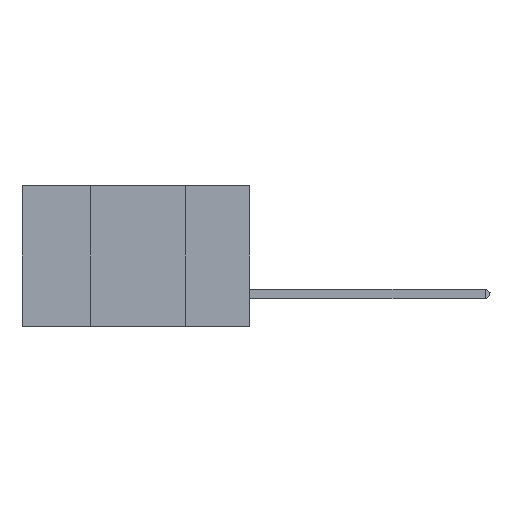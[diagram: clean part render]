
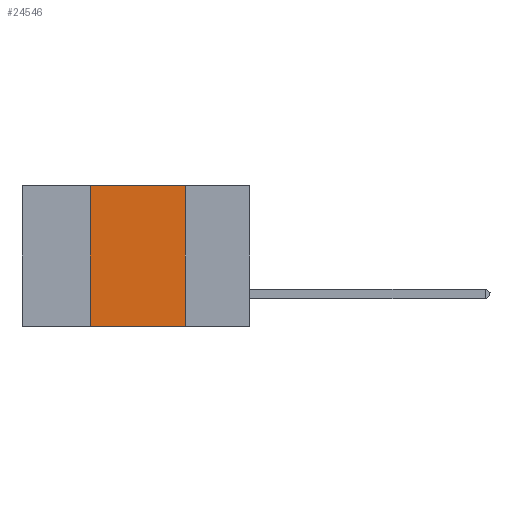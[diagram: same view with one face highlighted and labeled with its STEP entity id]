
A CAD part, left-side view. The second image highlights one B-rep face of the part: STEP entity #24546.
In plain terms, the highlighted planar face has unit normal (-1, 0, 0).
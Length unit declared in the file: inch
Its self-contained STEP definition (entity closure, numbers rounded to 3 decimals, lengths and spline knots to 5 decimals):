
#1889 = EDGE_CURVE ( 'NONE', #4909, #38383, #16010, .T. ) ;
#2787 = CARTESIAN_POINT ( 'NONE',  ( 0., 0.17, 0. ) ) ;
#4650 = EDGE_CURVE ( 'NONE', #35819, #38383, #13357, .T. ) ;
#4909 = VERTEX_POINT ( 'NONE', #5284 ) ;
#5284 = CARTESIAN_POINT ( 'NONE',  ( 0., 0.42, -0.37 ) ) ;
#7555 = ORIENTED_EDGE ( 'NONE', *, *, #4650, .F. ) ;
#8013 = VECTOR ( 'NONE', #19064, 39.37008 ) ;
#8151 = VECTOR ( 'NONE', #33141, 39.37008 ) ;
#10210 = CARTESIAN_POINT ( 'NONE',  ( 0., 0.42, 0. ) ) ;
#11245 = ORIENTED_EDGE ( 'NONE', *, *, #37221, .F. ) ;
#13078 = CARTESIAN_POINT ( 'NONE',  ( 0., 0.42, 0. ) ) ;
#13188 = ORIENTED_EDGE ( 'NONE', *, *, #33043, .F. ) ;
#13357 = LINE ( 'NONE', #21908, #24496 ) ;
#13408 = VECTOR ( 'NONE', #32555, 39.37008 ) ;
#16010 = LINE ( 'NONE', #27327, #8151 ) ;
#18001 = CARTESIAN_POINT ( 'NONE',  ( 0., 0.6, 0. ) ) ;
#18696 = EDGE_LOOP ( 'NONE', ( #7555, #13188, #11245, #33504 ) ) ;
#19064 = DIRECTION ( 'NONE',  ( 0., 0., 1. ) ) ;
#21165 = CARTESIAN_POINT ( 'NONE',  ( 0., 0.17, -0.37 ) ) ;
#21485 = PLANE ( 'NONE',  #35635 ) ;
#21908 = CARTESIAN_POINT ( 'NONE',  ( 0., 0.17, 0. ) ) ;
#24496 = VECTOR ( 'NONE', #30383, 39.37008 ) ;
#24546 = ADVANCED_FACE ( 'NONE', ( #25902 ), #21485, .F. ) ;
#25902 = FACE_OUTER_BOUND ( 'NONE', #18696, .T. ) ;
#27327 = CARTESIAN_POINT ( 'NONE',  ( 0., 0.6, -0.37 ) ) ;
#27612 = DIRECTION ( 'NONE',  ( 0., 0., -1. ) ) ;
#30383 = DIRECTION ( 'NONE',  ( 0., 0., -1. ) ) ;
#32555 = DIRECTION ( 'NONE',  ( 0., -1., 0. ) ) ;
#33043 = EDGE_CURVE ( 'NONE', #37898, #35819, #38565, .T. ) ;
#33141 = DIRECTION ( 'NONE',  ( 0., -1., 0. ) ) ;
#33504 = ORIENTED_EDGE ( 'NONE', *, *, #1889, .T. ) ;
#33818 = DIRECTION ( 'NONE',  ( 1., 0., 0. ) ) ;
#35635 = AXIS2_PLACEMENT_3D ( 'NONE', #36443, #33818, #27612 ) ;
#35819 = VERTEX_POINT ( 'NONE', #2787 ) ;
#36372 = LINE ( 'NONE', #13078, #8013 ) ;
#36443 = CARTESIAN_POINT ( 'NONE',  ( 0., 0.6, 0. ) ) ;
#37221 = EDGE_CURVE ( 'NONE', #4909, #37898, #36372, .T. ) ;
#37898 = VERTEX_POINT ( 'NONE', #10210 ) ;
#38383 = VERTEX_POINT ( 'NONE', #21165 ) ;
#38565 = LINE ( 'NONE', #18001, #13408 ) ;
